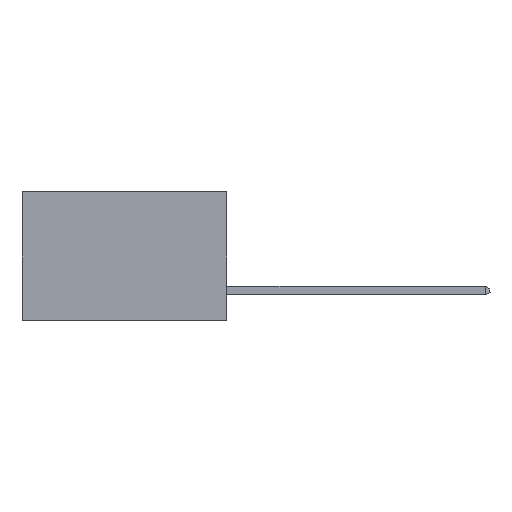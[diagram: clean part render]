
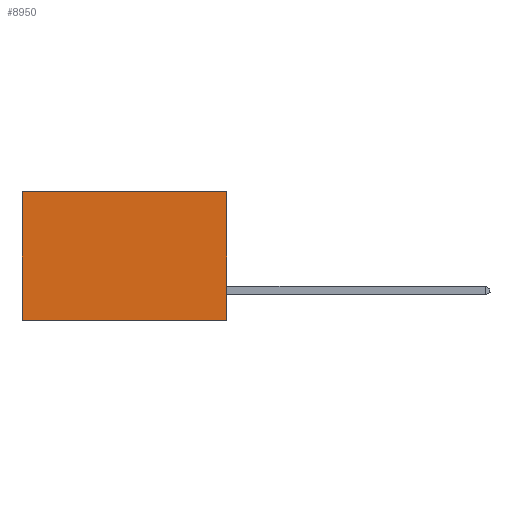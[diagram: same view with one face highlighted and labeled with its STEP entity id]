
A CAD part, left-side view. The second image highlights one B-rep face of the part: STEP entity #8950.
In plain terms, the highlighted planar face has unit normal (-1, 0, 0).
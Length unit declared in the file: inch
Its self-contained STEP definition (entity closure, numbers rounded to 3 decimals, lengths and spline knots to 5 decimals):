
#1815 = DIRECTION ( 'NONE',  ( 0., 1., 0. ) ) ;
#3060 = CARTESIAN_POINT ( 'NONE',  ( 0.277, 0.59, 0. ) ) ;
#4959 = ORIENTED_EDGE ( 'NONE', *, *, #5900, .T. ) ;
#5679 = LINE ( 'NONE', #16640, #31748 ) ;
#5900 = EDGE_CURVE ( 'NONE', #22485, #21784, #11601, .T. ) ;
#6881 = DIRECTION ( 'NONE',  ( 0., 1., 0. ) ) ;
#8950 = ADVANCED_FACE ( 'NONE', ( #9479 ), #15459, .F. ) ;
#9479 = FACE_OUTER_BOUND ( 'NONE', #30936, .T. ) ;
#11601 = LINE ( 'NONE', #30682, #31133 ) ;
#12083 = VECTOR ( 'NONE', #30475, 39.37008 ) ;
#12298 = CARTESIAN_POINT ( 'NONE',  ( 0.277, 0., 0. ) ) ;
#12849 = LINE ( 'NONE', #20654, #12083 ) ;
#13817 = ORIENTED_EDGE ( 'NONE', *, *, #24161, .F. ) ;
#14665 = LINE ( 'NONE', #26512, #20393 ) ;
#14783 = VERTEX_POINT ( 'NONE', #26869 ) ;
#14827 = AXIS2_PLACEMENT_3D ( 'NONE', #15558, #15279, #15239 ) ;
#14990 = CARTESIAN_POINT ( 'NONE',  ( 0.277, 0.59, -0.37 ) ) ;
#15131 = EDGE_CURVE ( 'NONE', #31580, #14783, #12849, .T. ) ;
#15239 = DIRECTION ( 'NONE',  ( 0., 0., -1. ) ) ;
#15279 = DIRECTION ( 'NONE',  ( 1., 0., 0. ) ) ;
#15459 = PLANE ( 'NONE',  #14827 ) ;
#15558 = CARTESIAN_POINT ( 'NONE',  ( 0.277, 0., -0.37 ) ) ;
#16640 = CARTESIAN_POINT ( 'NONE',  ( 0.277, 0., -0.37 ) ) ;
#19126 = ORIENTED_EDGE ( 'NONE', *, *, #22177, .T. ) ;
#20393 = VECTOR ( 'NONE', #6881, 39.37008 ) ;
#20654 = CARTESIAN_POINT ( 'NONE',  ( 0.277, 0., -0.37 ) ) ;
#21784 = VERTEX_POINT ( 'NONE', #14990 ) ;
#22177 = EDGE_CURVE ( 'NONE', #31580, #22485, #14665, .T. ) ;
#22485 = VERTEX_POINT ( 'NONE', #3060 ) ;
#24161 = EDGE_CURVE ( 'NONE', #14783, #21784, #5679, .T. ) ;
#26512 = CARTESIAN_POINT ( 'NONE',  ( 0.277, 0., 0. ) ) ;
#26869 = CARTESIAN_POINT ( 'NONE',  ( 0.277, 0., -0.37 ) ) ;
#27417 = ORIENTED_EDGE ( 'NONE', *, *, #15131, .F. ) ;
#30475 = DIRECTION ( 'NONE',  ( 0., 0., -1. ) ) ;
#30682 = CARTESIAN_POINT ( 'NONE',  ( 0.277, 0.59, -0.37 ) ) ;
#30827 = DIRECTION ( 'NONE',  ( 0., 0., -1. ) ) ;
#30936 = EDGE_LOOP ( 'NONE', ( #4959, #13817, #27417, #19126 ) ) ;
#31133 = VECTOR ( 'NONE', #30827, 39.37008 ) ;
#31580 = VERTEX_POINT ( 'NONE', #12298 ) ;
#31748 = VECTOR ( 'NONE', #1815, 39.37008 ) ;
